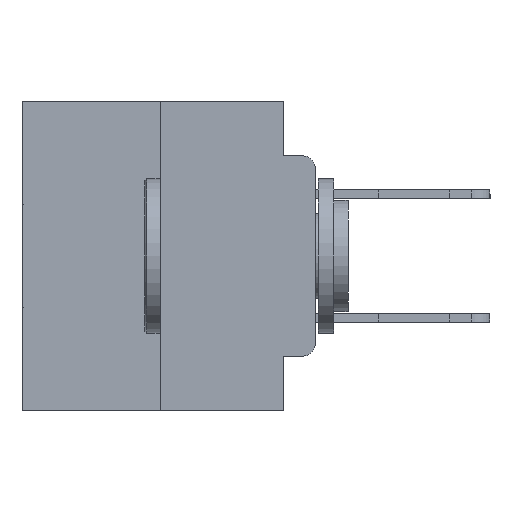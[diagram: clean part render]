
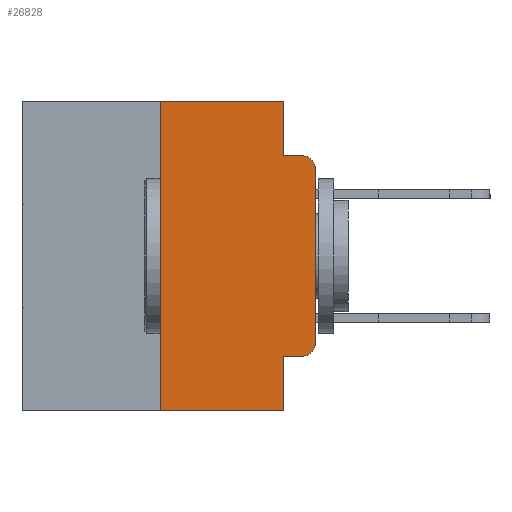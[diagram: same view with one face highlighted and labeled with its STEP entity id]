
A CAD part, left-side view. The second image highlights one B-rep face of the part: STEP entity #26828.
In plain terms, the highlighted planar face has unit normal (-1, 0, 0).
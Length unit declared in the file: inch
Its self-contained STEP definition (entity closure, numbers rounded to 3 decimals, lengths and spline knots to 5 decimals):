
#252 = VECTOR ( 'NONE', #18795, 39.37008 ) ;
#277 = CARTESIAN_POINT ( 'NONE',  ( 0., 0.02, -0.0885 ) ) ;
#600 = DIRECTION ( 'NONE',  ( 0., 0., 1. ) ) ;
#1396 = VECTOR ( 'NONE', #2221, 39.37008 ) ;
#1414 = FACE_OUTER_BOUND ( 'NONE', #27216, .T. ) ;
#1546 = VERTEX_POINT ( 'NONE', #27713 ) ;
#1921 = ORIENTED_EDGE ( 'NONE', *, *, #6250, .T. ) ;
#2221 = DIRECTION ( 'NONE',  ( 0., 0., 1. ) ) ;
#2578 = VERTEX_POINT ( 'NONE', #12821 ) ;
#2623 = LINE ( 'NONE', #27537, #7388 ) ;
#3031 = DIRECTION ( 'NONE',  ( 0., -1., 0. ) ) ;
#3578 = VECTOR ( 'NONE', #600, 39.37008 ) ;
#3666 = EDGE_CURVE ( 'NONE', #12878, #1546, #26885, .T. ) ;
#4421 = CARTESIAN_POINT ( 'NONE',  ( 0., 0., -0.3915 ) ) ;
#4590 = ORIENTED_EDGE ( 'NONE', *, *, #19103, .F. ) ;
#5211 = CIRCLE ( 'NONE', #8972, 0.02 ) ;
#5978 = DIRECTION ( 'NONE',  ( 0., 0., -1. ) ) ;
#6250 = EDGE_CURVE ( 'NONE', #28796, #2578, #10469, .T. ) ;
#6291 = VECTOR ( 'NONE', #5978, 39.37008 ) ;
#7388 = VECTOR ( 'NONE', #20861, 39.37008 ) ;
#8218 = AXIS2_PLACEMENT_3D ( 'NONE', #13217, #22312, #8704 ) ;
#8573 = ORIENTED_EDGE ( 'NONE', *, *, #25625, .T. ) ;
#8669 = DIRECTION ( 'NONE',  ( 0., -1., 0. ) ) ;
#8704 = DIRECTION ( 'NONE',  ( 0., 0., -1. ) ) ;
#8789 = AXIS2_PLACEMENT_3D ( 'NONE', #23497, #9954, #25728 ) ;
#8918 = ORIENTED_EDGE ( 'NONE', *, *, #3666, .F. ) ;
#8972 = AXIS2_PLACEMENT_3D ( 'NONE', #26521, #13081, #28724 ) ;
#9210 = CARTESIAN_POINT ( 'NONE',  ( 0., 0.051, -0.5 ) ) ;
#9618 = CARTESIAN_POINT ( 'NONE',  ( 0., 0.051, -0.4115 ) ) ;
#9954 = DIRECTION ( 'NONE',  ( -1., 0., 0. ) ) ;
#10038 = VERTEX_POINT ( 'NONE', #27251 ) ;
#10136 = EDGE_CURVE ( 'NONE', #23438, #25186, #2623, .T. ) ;
#10469 = LINE ( 'NONE', #21389, #3578 ) ;
#11444 = CARTESIAN_POINT ( 'NONE',  ( 0., 0.473, 0. ) ) ;
#11536 = VERTEX_POINT ( 'NONE', #16790 ) ;
#11880 = CARTESIAN_POINT ( 'NONE',  ( 0., 0.051, 0. ) ) ;
#12508 = CARTESIAN_POINT ( 'NONE',  ( 0., 0.25, 0. ) ) ;
#12519 = ORIENTED_EDGE ( 'NONE', *, *, #10136, .T. ) ;
#12821 = CARTESIAN_POINT ( 'NONE',  ( 0., 0., -0.1085 ) ) ;
#12878 = VERTEX_POINT ( 'NONE', #12508 ) ;
#12978 = EDGE_CURVE ( 'NONE', #10038, #25186, #25100, .T. ) ;
#13081 = DIRECTION ( 'NONE',  ( -1., 0., 0. ) ) ;
#13217 = CARTESIAN_POINT ( 'NONE',  ( 0., 0.473, 0. ) ) ;
#14171 = DIRECTION ( 'NONE',  ( 0., 0., -1. ) ) ;
#14285 = ORIENTED_EDGE ( 'NONE', *, *, #26517, .T. ) ;
#14515 = EDGE_CURVE ( 'NONE', #23438, #12878, #19833, .T. ) ;
#14855 = VECTOR ( 'NONE', #3031, 39.37008 ) ;
#16790 = CARTESIAN_POINT ( 'NONE',  ( 0., 0.051, -0.0885 ) ) ;
#16860 = CARTESIAN_POINT ( 'NONE',  ( 0., 0.051, -0.0885 ) ) ;
#17047 = CIRCLE ( 'NONE', #8789, 0.02 ) ;
#17409 = CARTESIAN_POINT ( 'NONE',  ( 0., 0.051, 0. ) ) ;
#17589 = EDGE_CURVE ( 'NONE', #1546, #11536, #18516, .T. ) ;
#18516 = LINE ( 'NONE', #11880, #23739 ) ;
#18601 = ORIENTED_EDGE ( 'NONE', *, *, #12978, .F. ) ;
#18781 = LINE ( 'NONE', #9618, #252 ) ;
#18795 = DIRECTION ( 'NONE',  ( 0., -1., 0. ) ) ;
#19103 = EDGE_CURVE ( 'NONE', #11536, #25955, #21557, .T. ) ;
#19833 = LINE ( 'NONE', #29396, #1396 ) ;
#20077 = PLANE ( 'NONE',  #8218 ) ;
#20308 = VECTOR ( 'NONE', #8669, 39.37008 ) ;
#20861 = DIRECTION ( 'NONE',  ( 0., -1., 0. ) ) ;
#21144 = VERTEX_POINT ( 'NONE', #28472 ) ;
#21389 = CARTESIAN_POINT ( 'NONE',  ( 0., 0., 0. ) ) ;
#21557 = LINE ( 'NONE', #16860, #14855 ) ;
#22312 = DIRECTION ( 'NONE',  ( 1., 0., 0. ) ) ;
#22421 = ORIENTED_EDGE ( 'NONE', *, *, #14515, .F. ) ;
#23183 = CARTESIAN_POINT ( 'NONE',  ( 0., 0.25, -0.5 ) ) ;
#23438 = VERTEX_POINT ( 'NONE', #23183 ) ;
#23460 = ORIENTED_EDGE ( 'NONE', *, *, #17589, .F. ) ;
#23497 = CARTESIAN_POINT ( 'NONE',  ( 0., 0.02, -0.1085 ) ) ;
#23739 = VECTOR ( 'NONE', #14171, 39.37008 ) ;
#24516 = ORIENTED_EDGE ( 'NONE', *, *, #27058, .T. ) ;
#25100 = LINE ( 'NONE', #17409, #6291 ) ;
#25186 = VERTEX_POINT ( 'NONE', #9210 ) ;
#25625 = EDGE_CURVE ( 'NONE', #21144, #28796, #5211, .T. ) ;
#25728 = DIRECTION ( 'NONE',  ( 0., 0., -1. ) ) ;
#25955 = VERTEX_POINT ( 'NONE', #277 ) ;
#26517 = EDGE_CURVE ( 'NONE', #2578, #25955, #17047, .T. ) ;
#26521 = CARTESIAN_POINT ( 'NONE',  ( 0., 0.02, -0.3915 ) ) ;
#26828 = ADVANCED_FACE ( 'NONE', ( #1414 ), #20077, .F. ) ;
#26885 = LINE ( 'NONE', #11444, #20308 ) ;
#27058 = EDGE_CURVE ( 'NONE', #10038, #21144, #18781, .T. ) ;
#27216 = EDGE_LOOP ( 'NONE', ( #1921, #14285, #4590, #23460, #8918, #22421, #12519, #18601, #24516, #8573 ) ) ;
#27251 = CARTESIAN_POINT ( 'NONE',  ( 0., 0.051, -0.4115 ) ) ;
#27537 = CARTESIAN_POINT ( 'NONE',  ( 0., 0.473, -0.5 ) ) ;
#27713 = CARTESIAN_POINT ( 'NONE',  ( 0., 0.051, 0. ) ) ;
#28472 = CARTESIAN_POINT ( 'NONE',  ( 0., 0.02, -0.4115 ) ) ;
#28724 = DIRECTION ( 'NONE',  ( 0., 0., -1. ) ) ;
#28796 = VERTEX_POINT ( 'NONE', #4421 ) ;
#29396 = CARTESIAN_POINT ( 'NONE',  ( 0., 0.25, 0. ) ) ;
